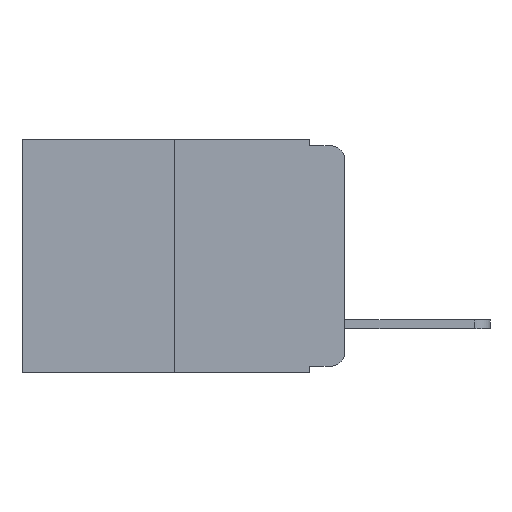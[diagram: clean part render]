
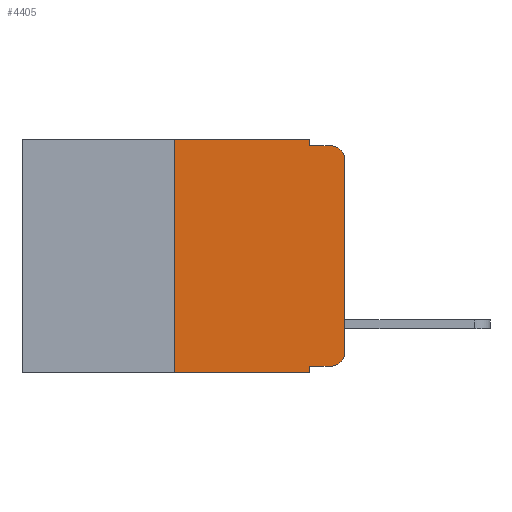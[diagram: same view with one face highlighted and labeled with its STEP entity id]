
A CAD part, left-side view. The second image highlights one B-rep face of the part: STEP entity #4405.
In plain terms, the highlighted planar face has unit normal (-1, 0, 0).
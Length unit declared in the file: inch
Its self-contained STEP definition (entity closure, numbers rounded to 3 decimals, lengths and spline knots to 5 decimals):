
#81 = VECTOR ( 'NONE', #13419, 39.37008 ) ;
#274 = EDGE_CURVE ( 'NONE', #2913, #8924, #2750, .T. ) ;
#372 = VERTEX_POINT ( 'NONE', #15721 ) ;
#447 = VECTOR ( 'NONE', #8719, 39.37008 ) ;
#612 = VECTOR ( 'NONE', #13725, 39.37008 ) ;
#671 = AXIS2_PLACEMENT_3D ( 'NONE', #1484, #10231, #2927 ) ;
#757 = CARTESIAN_POINT ( 'NONE',  ( 0., 0.051, -0.01 ) ) ;
#880 = VERTEX_POINT ( 'NONE', #2982 ) ;
#1176 = ORIENTED_EDGE ( 'NONE', *, *, #2235, .F. ) ;
#1243 = EDGE_CURVE ( 'NONE', #5395, #372, #10550, .T. ) ;
#1455 = CARTESIAN_POINT ( 'NONE',  ( 0., 0., 0. ) ) ;
#1484 = CARTESIAN_POINT ( 'NONE',  ( 0., 0.02, -0.03 ) ) ;
#1494 = EDGE_CURVE ( 'NONE', #5395, #8924, #3575, .T. ) ;
#2013 = CARTESIAN_POINT ( 'NONE',  ( 0., 0.051, -0.01 ) ) ;
#2235 = EDGE_CURVE ( 'NONE', #2522, #12502, #8455, .T. ) ;
#2247 = DIRECTION ( 'NONE',  ( 0., -1., 0. ) ) ;
#2307 = CARTESIAN_POINT ( 'NONE',  ( 0., 0.473, -0.343 ) ) ;
#2522 = VERTEX_POINT ( 'NONE', #8725 ) ;
#2563 = CIRCLE ( 'NONE', #14304, 0.02 ) ;
#2585 = ORIENTED_EDGE ( 'NONE', *, *, #5834, .T. ) ;
#2750 = LINE ( 'NONE', #2791, #8592 ) ;
#2791 = CARTESIAN_POINT ( 'NONE',  ( 0., 0.051, 0. ) ) ;
#2886 = VECTOR ( 'NONE', #11839, 39.37008 ) ;
#2913 = VERTEX_POINT ( 'NONE', #14439 ) ;
#2927 = DIRECTION ( 'NONE',  ( 0., 0., -1. ) ) ;
#2982 = CARTESIAN_POINT ( 'NONE',  ( 0., 0., -0.313 ) ) ;
#3049 = CARTESIAN_POINT ( 'NONE',  ( 0., 0.473, 0. ) ) ;
#3171 = EDGE_CURVE ( 'NONE', #12502, #9492, #11346, .T. ) ;
#3547 = ORIENTED_EDGE ( 'NONE', *, *, #6621, .T. ) ;
#3575 = LINE ( 'NONE', #2307, #12739 ) ;
#4334 = LINE ( 'NONE', #1455, #612 ) ;
#4398 = DIRECTION ( 'NONE',  ( 0., 0., -1. ) ) ;
#4405 = ADVANCED_FACE ( 'NONE', ( #13320 ), #10337, .F. ) ;
#4504 = ORIENTED_EDGE ( 'NONE', *, *, #1243, .F. ) ;
#4703 = EDGE_LOOP ( 'NONE', ( #3547, #2585, #5181, #1176, #12810, #4504, #8733, #11930, #9898, #6510 ) ) ;
#4761 = CARTESIAN_POINT ( 'NONE',  ( 0., 0.051, -0.333 ) ) ;
#5181 = ORIENTED_EDGE ( 'NONE', *, *, #3171, .F. ) ;
#5395 = VERTEX_POINT ( 'NONE', #14894 ) ;
#5531 = VECTOR ( 'NONE', #12264, 39.37008 ) ;
#5834 = EDGE_CURVE ( 'NONE', #9426, #9492, #13975, .T. ) ;
#6510 = ORIENTED_EDGE ( 'NONE', *, *, #14646, .T. ) ;
#6621 = EDGE_CURVE ( 'NONE', #880, #9426, #4334, .T. ) ;
#6834 = DIRECTION ( 'NONE',  ( -1., 0., 0. ) ) ;
#7008 = CARTESIAN_POINT ( 'NONE',  ( 0., 0.02, -0.333 ) ) ;
#7242 = LINE ( 'NONE', #13364, #81 ) ;
#8210 = CARTESIAN_POINT ( 'NONE',  ( 0., 0.02, -0.01 ) ) ;
#8455 = LINE ( 'NONE', #14206, #13908 ) ;
#8592 = VECTOR ( 'NONE', #15683, 39.37008 ) ;
#8640 = AXIS2_PLACEMENT_3D ( 'NONE', #3049, #11517, #4398 ) ;
#8719 = DIRECTION ( 'NONE',  ( 0., 0., 1. ) ) ;
#8725 = CARTESIAN_POINT ( 'NONE',  ( 0., 0.051, 0. ) ) ;
#8733 = ORIENTED_EDGE ( 'NONE', *, *, #1494, .T. ) ;
#8924 = VERTEX_POINT ( 'NONE', #13067 ) ;
#9426 = VERTEX_POINT ( 'NONE', #13883 ) ;
#9492 = VERTEX_POINT ( 'NONE', #8210 ) ;
#9898 = ORIENTED_EDGE ( 'NONE', *, *, #15448, .T. ) ;
#10231 = DIRECTION ( 'NONE',  ( -1., 0., 0. ) ) ;
#10337 = PLANE ( 'NONE',  #8640 ) ;
#10550 = LINE ( 'NONE', #11050, #447 ) ;
#11050 = CARTESIAN_POINT ( 'NONE',  ( 0., 0.25, 0. ) ) ;
#11346 = LINE ( 'NONE', #2013, #5531 ) ;
#11517 = DIRECTION ( 'NONE',  ( 1., 0., 0. ) ) ;
#11839 = DIRECTION ( 'NONE',  ( 0., -1., 0. ) ) ;
#11930 = ORIENTED_EDGE ( 'NONE', *, *, #274, .F. ) ;
#12172 = LINE ( 'NONE', #4761, #2886 ) ;
#12264 = DIRECTION ( 'NONE',  ( 0., -1., 0. ) ) ;
#12280 = VERTEX_POINT ( 'NONE', #7008 ) ;
#12502 = VERTEX_POINT ( 'NONE', #757 ) ;
#12739 = VECTOR ( 'NONE', #2247, 39.37008 ) ;
#12810 = ORIENTED_EDGE ( 'NONE', *, *, #14017, .F. ) ;
#13067 = CARTESIAN_POINT ( 'NONE',  ( 0., 0.051, -0.343 ) ) ;
#13320 = FACE_OUTER_BOUND ( 'NONE', #4703, .T. ) ;
#13364 = CARTESIAN_POINT ( 'NONE',  ( 0., 0.473, 0. ) ) ;
#13419 = DIRECTION ( 'NONE',  ( 0., -1., 0. ) ) ;
#13725 = DIRECTION ( 'NONE',  ( 0., 0., 1. ) ) ;
#13767 = CARTESIAN_POINT ( 'NONE',  ( 0., 0.02, -0.313 ) ) ;
#13883 = CARTESIAN_POINT ( 'NONE',  ( 0., 0., -0.03 ) ) ;
#13908 = VECTOR ( 'NONE', #14166, 39.37008 ) ;
#13975 = CIRCLE ( 'NONE', #671, 0.02 ) ;
#14017 = EDGE_CURVE ( 'NONE', #372, #2522, #7242, .T. ) ;
#14166 = DIRECTION ( 'NONE',  ( 0., 0., -1. ) ) ;
#14206 = CARTESIAN_POINT ( 'NONE',  ( 0., 0.051, 0. ) ) ;
#14304 = AXIS2_PLACEMENT_3D ( 'NONE', #13767, #6834, #14899 ) ;
#14439 = CARTESIAN_POINT ( 'NONE',  ( 0., 0.051, -0.333 ) ) ;
#14646 = EDGE_CURVE ( 'NONE', #12280, #880, #2563, .T. ) ;
#14894 = CARTESIAN_POINT ( 'NONE',  ( 0., 0.25, -0.343 ) ) ;
#14899 = DIRECTION ( 'NONE',  ( 0., 0., -1. ) ) ;
#15448 = EDGE_CURVE ( 'NONE', #2913, #12280, #12172, .T. ) ;
#15683 = DIRECTION ( 'NONE',  ( 0., 0., -1. ) ) ;
#15721 = CARTESIAN_POINT ( 'NONE',  ( 0., 0.25, 0. ) ) ;
